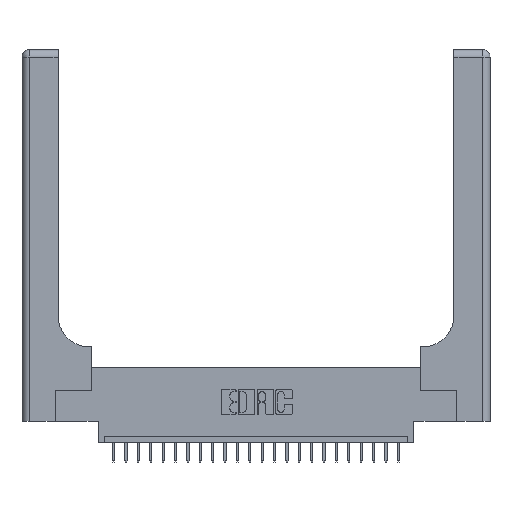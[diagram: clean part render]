
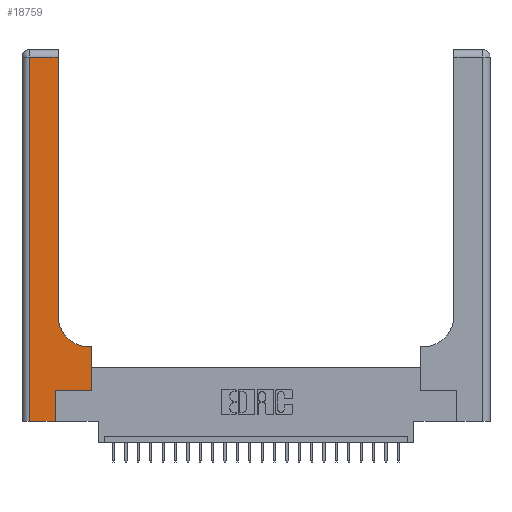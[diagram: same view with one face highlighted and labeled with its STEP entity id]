
A CAD part, top view. The second image highlights one B-rep face of the part: STEP entity #18759.
In plain terms, the highlighted planar face has unit normal (0, 0, 1).
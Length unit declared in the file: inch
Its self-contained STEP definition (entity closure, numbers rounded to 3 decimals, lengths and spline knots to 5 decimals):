
#303 = CARTESIAN_POINT ( 'NONE',  ( 0.2915, 3., 0.37 ) ) ;
#326 = VECTOR ( 'NONE', #4033, 39.37008 ) ;
#715 = EDGE_CURVE ( 'NONE', #16757, #20650, #18679, .T. ) ;
#1095 = DIRECTION ( 'NONE',  ( -1., 0., 0. ) ) ;
#1358 = EDGE_CURVE ( 'NONE', #25363, #23528, #14910, .T. ) ;
#1880 = DIRECTION ( 'NONE',  ( 0., 1., 0. ) ) ;
#2312 = ORIENTED_EDGE ( 'NONE', *, *, #1358, .T. ) ;
#2680 = ORIENTED_EDGE ( 'NONE', *, *, #18063, .T. ) ;
#4033 = DIRECTION ( 'NONE',  ( 0., 1., 0. ) ) ;
#4373 = DIRECTION ( 'NONE',  ( -1., 0., 0. ) ) ;
#4781 = VERTEX_POINT ( 'NONE', #25412 ) ;
#5008 = VECTOR ( 'NONE', #1880, 39.37008 ) ;
#5102 = VECTOR ( 'NONE', #7060, 39.37008 ) ;
#5406 = EDGE_CURVE ( 'NONE', #20650, #25235, #13150, .T. ) ;
#7060 = DIRECTION ( 'NONE',  ( 0., 1., 0. ) ) ;
#7092 = FACE_OUTER_BOUND ( 'NONE', #21116, .T. ) ;
#8583 = VERTEX_POINT ( 'NONE', #25397 ) ;
#9732 = ORIENTED_EDGE ( 'NONE', *, *, #17522, .T. ) ;
#9776 = DIRECTION ( 'NONE',  ( 1., 0., 0. ) ) ;
#9868 = CARTESIAN_POINT ( 'NONE',  ( 0.269, 0.25, 0.37 ) ) ;
#9898 = CARTESIAN_POINT ( 'NONE',  ( 0.5585, 0.25, 0.37 ) ) ;
#10631 = DIRECTION ( 'NONE',  ( 0., -1., 0. ) ) ;
#10654 = EDGE_CURVE ( 'NONE', #23528, #25673, #12449, .T. ) ;
#10738 = VECTOR ( 'NONE', #9776, 39.37008 ) ;
#11734 = AXIS2_PLACEMENT_3D ( 'NONE', #17304, #25064, #17397 ) ;
#11748 = CARTESIAN_POINT ( 'NONE',  ( 0.269, 0., 0.37 ) ) ;
#12449 = LINE ( 'NONE', #13014, #17469 ) ;
#13014 = CARTESIAN_POINT ( 'NONE',  ( 0., 0., 0.37 ) ) ;
#13029 = PLANE ( 'NONE',  #21826 ) ;
#13150 = LINE ( 'NONE', #303, #5008 ) ;
#13663 = VECTOR ( 'NONE', #4373, 39.37008 ) ;
#13970 = LINE ( 'NONE', #16375, #13663 ) ;
#14499 = EDGE_CURVE ( 'NONE', #8583, #20195, #19491, .T. ) ;
#14644 = ORIENTED_EDGE ( 'NONE', *, *, #10654, .T. ) ;
#14664 = LINE ( 'NONE', #11748, #326 ) ;
#14910 = LINE ( 'NONE', #20350, #23372 ) ;
#15087 = CARTESIAN_POINT ( 'NONE',  ( 0.06, 2.94, 0.37 ) ) ;
#16020 = ORIENTED_EDGE ( 'NONE', *, *, #22775, .T. ) ;
#16375 = CARTESIAN_POINT ( 'NONE',  ( 0., 2.94, 0.37 ) ) ;
#16517 = LINE ( 'NONE', #19494, #21213 ) ;
#16757 = VERTEX_POINT ( 'NONE', #23068 ) ;
#17304 = CARTESIAN_POINT ( 'NONE',  ( 0.5415, 0.85, 0.37 ) ) ;
#17397 = DIRECTION ( 'NONE',  ( 1., 0., 0. ) ) ;
#17469 = VECTOR ( 'NONE', #25529, 39.37008 ) ;
#17522 = EDGE_CURVE ( 'NONE', #25673, #8583, #14664, .T. ) ;
#17602 = CARTESIAN_POINT ( 'NONE',  ( 0.06, 0., 0.37 ) ) ;
#17671 = DIRECTION ( 'NONE',  ( -1., 0., 0. ) ) ;
#18063 = EDGE_CURVE ( 'NONE', #4781, #16757, #16517, .T. ) ;
#18649 = EDGE_CURVE ( 'NONE', #25235, #25363, #13970, .T. ) ;
#18679 = CIRCLE ( 'NONE', #11734, 0.25 ) ;
#18759 = ADVANCED_FACE ( 'NONE', ( #7092 ), #13029, .F. ) ;
#18875 = DIRECTION ( 'NONE',  ( 0., 0., -1. ) ) ;
#19192 = CARTESIAN_POINT ( 'NONE',  ( 0.5585, 0.25, 0.37 ) ) ;
#19319 = CARTESIAN_POINT ( 'NONE',  ( 0.2915, 0.85, 0.37 ) ) ;
#19491 = LINE ( 'NONE', #9868, #10738 ) ;
#19494 = CARTESIAN_POINT ( 'NONE',  ( 0.2915, 0.6, 0.37 ) ) ;
#19517 = LINE ( 'NONE', #19192, #5102 ) ;
#19810 = ORIENTED_EDGE ( 'NONE', *, *, #18649, .T. ) ;
#20195 = VERTEX_POINT ( 'NONE', #9898 ) ;
#20350 = CARTESIAN_POINT ( 'NONE',  ( 0.06, 3., 0.37 ) ) ;
#20650 = VERTEX_POINT ( 'NONE', #19319 ) ;
#21116 = EDGE_LOOP ( 'NONE', ( #23840, #19810, #2312, #14644, #9732, #23188, #16020, #2680, #22196 ) ) ;
#21213 = VECTOR ( 'NONE', #17671, 39.37008 ) ;
#21639 = CARTESIAN_POINT ( 'NONE',  ( 0.269, 0., 0.37 ) ) ;
#21826 = AXIS2_PLACEMENT_3D ( 'NONE', #22679, #18875, #1095 ) ;
#22196 = ORIENTED_EDGE ( 'NONE', *, *, #715, .T. ) ;
#22679 = CARTESIAN_POINT ( 'NONE',  ( 0., 3., 0.37 ) ) ;
#22775 = EDGE_CURVE ( 'NONE', #20195, #4781, #19517, .T. ) ;
#22791 = CARTESIAN_POINT ( 'NONE',  ( 0.2915, 2.94, 0.37 ) ) ;
#23068 = CARTESIAN_POINT ( 'NONE',  ( 0.5415, 0.6, 0.37 ) ) ;
#23188 = ORIENTED_EDGE ( 'NONE', *, *, #14499, .T. ) ;
#23372 = VECTOR ( 'NONE', #10631, 39.37008 ) ;
#23528 = VERTEX_POINT ( 'NONE', #17602 ) ;
#23840 = ORIENTED_EDGE ( 'NONE', *, *, #5406, .T. ) ;
#25064 = DIRECTION ( 'NONE',  ( 0., 0., -1. ) ) ;
#25235 = VERTEX_POINT ( 'NONE', #22791 ) ;
#25363 = VERTEX_POINT ( 'NONE', #15087 ) ;
#25397 = CARTESIAN_POINT ( 'NONE',  ( 0.269, 0.25, 0.37 ) ) ;
#25412 = CARTESIAN_POINT ( 'NONE',  ( 0.5585, 0.6, 0.37 ) ) ;
#25529 = DIRECTION ( 'NONE',  ( 1., 0., 0. ) ) ;
#25673 = VERTEX_POINT ( 'NONE', #21639 ) ;
